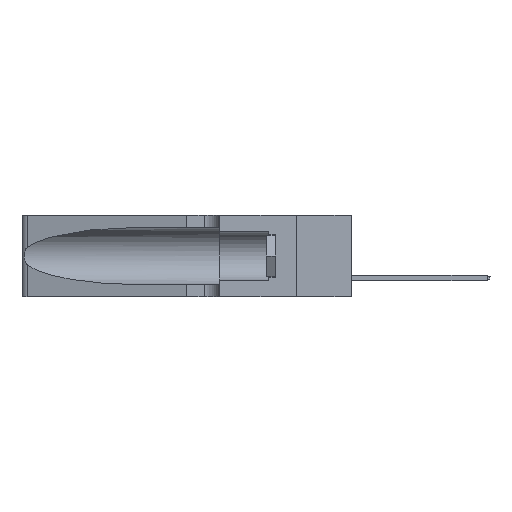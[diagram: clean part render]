
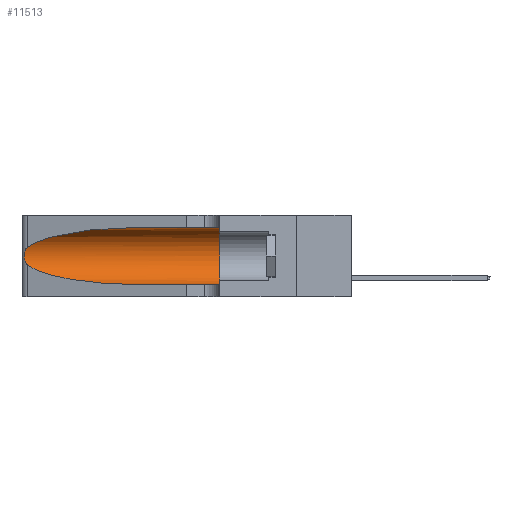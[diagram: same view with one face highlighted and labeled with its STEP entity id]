
A CAD part, left-side view. The second image highlights one B-rep face of the part: STEP entity #11513.
In plain terms, the highlighted cylindrical face has radius 3.308 mm (diameter 6.617 mm), a partial arc.
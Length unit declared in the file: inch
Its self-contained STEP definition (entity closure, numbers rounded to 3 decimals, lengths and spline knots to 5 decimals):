
#142 = CARTESIAN_POINT ( 'NONE',  ( 0.1305, 0.35, 0.05475 ) ) ;
#295 = CARTESIAN_POINT ( 'NONE',  ( 0.25639, 1.23186, 0.15144 ) ) ;
#379 = CARTESIAN_POINT ( 'NONE',  ( 0.26017, 1.23833, 0.17102 ) ) ;
#645 = CARTESIAN_POINT ( 'NONE',  ( 0.25487, 1.22718, 0.14631 ) ) ;
#1010 = AXIS2_PLACEMENT_3D ( 'NONE', #14096, #15982, #17983 ) ;
#1117 = CARTESIAN_POINT ( 'NONE',  ( 0.1305, 0.72297, 0.05475 ) ) ;
#1410 = EDGE_CURVE ( 'NONE', #16538, #9235, #18909, .T. ) ;
#1528 = EDGE_CURVE ( 'NONE', #21286, #14615, #16008, .T. ) ;
#2460 = CARTESIAN_POINT ( 'NONE',  ( 0.26018, 1.23835, 0.19895 ) ) ;
#3097 = CARTESIAN_POINT ( 'NONE',  ( 0.1305, 0.35, 0.31525 ) ) ;
#4694 = EDGE_LOOP ( 'NONE', ( #12690, #11040, #25860, #19644, #13336, #13640 ) ) ;
#5719 = FACE_OUTER_BOUND ( 'NONE', #4694, .T. ) ;
#6001 = CIRCLE ( 'NONE', #1010, 0.13025 ) ;
#6162 = EDGE_CURVE ( 'NONE', #9235, #15660, #18323, .T. ) ;
#6524 = CARTESIAN_POINT ( 'NONE',  ( 0.25555, 1.22994, 0.2215 ) ) ;
#7073 = B_SPLINE_CURVE_WITH_KNOTS ( 'NONE', 3,
 ( #24254, #6524, #21097, #23302, #14896, #2460, #12843, #15079, #379, #8612, #19085, #295, #16955, #14990 ),
 .UNSPECIFIED., .F., .F.,
 ( 4, 2, 2, 2, 2, 2, 4 ),
 ( 0., 0.00027, 0.00053, 0.00107, 0.0016, 0.00187, 0.00214 ),
 .UNSPECIFIED. ) ;
#7227 = VECTOR ( 'NONE', #7465, 39.37008 ) ;
#7465 = DIRECTION ( 'NONE',  ( 0., -1., 0. ) ) ;
#8302 = CYLINDRICAL_SURFACE ( 'NONE', #23363, 0.13025 ) ;
#8612 = CARTESIAN_POINT ( 'NONE',  ( 0.25856, 1.23593, 0.16098 ) ) ;
#8701 = VERTEX_POINT ( 'NONE', #20648 ) ;
#9235 = VERTEX_POINT ( 'NONE', #24477 ) ;
#9265 = CARTESIAN_POINT ( 'NONE',  ( 0.18966, 0.96281, 0.31525 ) ) ;
#9552 = CARTESIAN_POINT ( 'NONE',  ( 0.25487, 1.22718, 0.14631 ) ) ;
#10694 = CARTESIAN_POINT ( 'NONE',  ( 0.1305, 1.61858, 0.185 ) ) ;
#11040 = ORIENTED_EDGE ( 'NONE', *, *, #21405, .T. ) ;
#11513 = ADVANCED_FACE ( 'NONE', ( #5719 ), #8302, .F. ) ;
#11952 =( BOUNDED_CURVE ( )  B_SPLINE_CURVE ( 3, ( #23790, #9265, #21573, #13231 ),
 .UNSPECIFIED., .F., .F. ) 
 B_SPLINE_CURVE_WITH_KNOTS ( ( 4, 4 ),
 ( 1.5708, 2.84003 ),
 .UNSPECIFIED. ) 
 CURVE ( )  GEOMETRIC_REPRESENTATION_ITEM ( )  RATIONAL_B_SPLINE_CURVE ( ( 1., 0.87, 0.87, 1. ) ) 
 REPRESENTATION_ITEM ( '' )  );
#12204 = DIRECTION ( 'NONE',  ( 0., -1., 0. ) ) ;
#12646 = EDGE_CURVE ( 'NONE', #14615, #15660, #6001, .T. ) ;
#12690 = ORIENTED_EDGE ( 'NONE', *, *, #15738, .T. ) ;
#12843 = CARTESIAN_POINT ( 'NONE',  ( 0.26075, 1.23896, 0.19203 ) ) ;
#13231 = CARTESIAN_POINT ( 'NONE',  ( 0.25487, 1.22718, 0.22369 ) ) ;
#13336 = ORIENTED_EDGE ( 'NONE', *, *, #12646, .F. ) ;
#13507 = VECTOR ( 'NONE', #12204, 39.37008 ) ;
#13596 = CARTESIAN_POINT ( 'NONE',  ( 0.1305, 1.61858, 0.31525 ) ) ;
#13640 = ORIENTED_EDGE ( 'NONE', *, *, #1528, .F. ) ;
#14096 = CARTESIAN_POINT ( 'NONE',  ( 0.1305, 0.35, 0.185 ) ) ;
#14615 = VERTEX_POINT ( 'NONE', #3097 ) ;
#14689 = CARTESIAN_POINT ( 'NONE',  ( 0.1305, 0.72297, 0.31525 ) ) ;
#14896 = CARTESIAN_POINT ( 'NONE',  ( 0.25854, 1.2359, 0.20912 ) ) ;
#14990 = CARTESIAN_POINT ( 'NONE',  ( 0.25487, 1.22718, 0.14631 ) ) ;
#15079 = CARTESIAN_POINT ( 'NONE',  ( 0.26075, 1.23896, 0.178 ) ) ;
#15660 = VERTEX_POINT ( 'NONE', #142 ) ;
#15738 = EDGE_CURVE ( 'NONE', #21286, #8701, #11952, .T. ) ;
#15982 = DIRECTION ( 'NONE',  ( 0., 1., 0. ) ) ;
#16008 = LINE ( 'NONE', #13596, #7227 ) ;
#16538 = VERTEX_POINT ( 'NONE', #645 ) ;
#16940 = DIRECTION ( 'NONE',  ( 0., 0., -1. ) ) ;
#16955 = CARTESIAN_POINT ( 'NONE',  ( 0.25555, 1.22993, 0.14849 ) ) ;
#17983 = DIRECTION ( 'NONE',  ( 0., 0., 1. ) ) ;
#18323 = LINE ( 'NONE', #18528, #13507 ) ;
#18528 = CARTESIAN_POINT ( 'NONE',  ( 0.1305, 1.61858, 0.05475 ) ) ;
#18909 =( BOUNDED_CURVE ( )  B_SPLINE_CURVE ( 3, ( #9552, #19574, #21844, #1117 ),
 .UNSPECIFIED., .F., .T. ) 
 B_SPLINE_CURVE_WITH_KNOTS ( ( 4, 4 ),
 ( 3.44316, 4.71239 ),
 .UNSPECIFIED. ) 
 CURVE ( )  GEOMETRIC_REPRESENTATION_ITEM ( )  RATIONAL_B_SPLINE_CURVE ( ( 1., 0.87, 0.87, 1. ) ) 
 REPRESENTATION_ITEM ( '' )  );
#19085 = CARTESIAN_POINT ( 'NONE',  ( 0.25789, 1.23486, 0.15765 ) ) ;
#19574 = CARTESIAN_POINT ( 'NONE',  ( 0.2373, 1.15595, 0.08982 ) ) ;
#19644 = ORIENTED_EDGE ( 'NONE', *, *, #6162, .T. ) ;
#20648 = CARTESIAN_POINT ( 'NONE',  ( 0.25487, 1.22718, 0.22369 ) ) ;
#21097 = CARTESIAN_POINT ( 'NONE',  ( 0.25639, 1.23184, 0.21858 ) ) ;
#21286 = VERTEX_POINT ( 'NONE', #14689 ) ;
#21405 = EDGE_CURVE ( 'NONE', #8701, #16538, #7073, .T. ) ;
#21573 = CARTESIAN_POINT ( 'NONE',  ( 0.2373, 1.15595, 0.28018 ) ) ;
#21844 = CARTESIAN_POINT ( 'NONE',  ( 0.18966, 0.96281, 0.05475 ) ) ;
#23302 = CARTESIAN_POINT ( 'NONE',  ( 0.25787, 1.23484, 0.2124 ) ) ;
#23363 = AXIS2_PLACEMENT_3D ( 'NONE', #10694, #25316, #16940 ) ;
#23790 = CARTESIAN_POINT ( 'NONE',  ( 0.1305, 0.72297, 0.31525 ) ) ;
#24254 = CARTESIAN_POINT ( 'NONE',  ( 0.25487, 1.22718, 0.22369 ) ) ;
#24477 = CARTESIAN_POINT ( 'NONE',  ( 0.1305, 0.72297, 0.05475 ) ) ;
#25316 = DIRECTION ( 'NONE',  ( 0., -1., 0. ) ) ;
#25860 = ORIENTED_EDGE ( 'NONE', *, *, #1410, .T. ) ;
